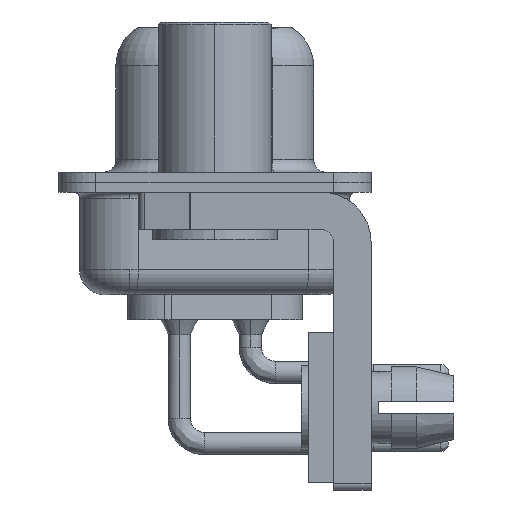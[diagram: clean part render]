
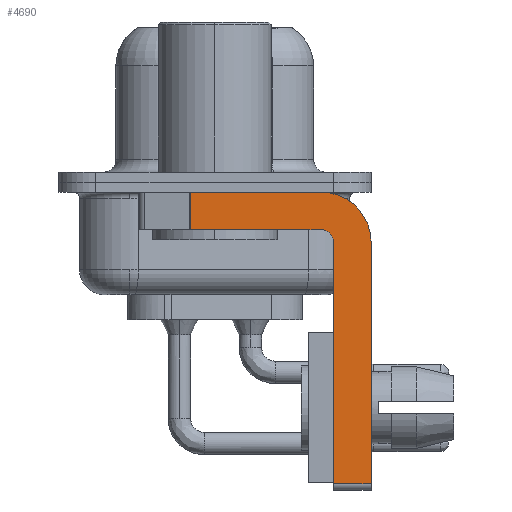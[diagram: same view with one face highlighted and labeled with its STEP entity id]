
A CAD part, left-side view. The second image highlights one B-rep face of the part: STEP entity #4690.
In plain terms, the highlighted planar face has unit normal (-1, 0, 0).
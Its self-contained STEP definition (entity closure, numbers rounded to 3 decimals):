
#132 = CARTESIAN_POINT ( 'NONE',  ( -2.9, -4.25, -1.9 ) ) ;
#850 = CARTESIAN_POINT ( 'NONE',  ( -2.9, -4.25, -1.9 ) ) ;
#1033 = DIRECTION ( 'NONE',  ( -1., 0., 0. ) ) ;
#1676 = LINE ( 'NONE', #17092, #6828 ) ;
#1708 = LINE ( 'NONE', #9999, #8234 ) ;
#1746 = DIRECTION ( 'NONE',  ( 1., 0., 0. ) ) ;
#1796 = CARTESIAN_POINT ( 'NONE',  ( -2.9, 0.978, -1.9 ) ) ;
#1817 = CARTESIAN_POINT ( 'NONE',  ( -2.9, -4.25, -2.4 ) ) ;
#2197 = LINE ( 'NONE', #16255, #24327 ) ;
#2657 = CARTESIAN_POINT ( 'NONE',  ( -2.9, -4.25, -2.4 ) ) ;
#2817 = ORIENTED_EDGE ( 'NONE', *, *, #11641, .F. ) ;
#3050 = EDGE_CURVE ( 'NONE', #20689, #22344, #12436, .T. ) ;
#3237 = LINE ( 'NONE', #25638, #19055 ) ;
#3828 = DIRECTION ( 'NONE',  ( 0., 0., -1. ) ) ;
#3836 = CARTESIAN_POINT ( 'NONE',  ( -2.9, -4.25, -0.4 ) ) ;
#3921 = PLANE ( 'NONE',  #12846 ) ;
#4125 = VERTEX_POINT ( 'NONE', #23902 ) ;
#4253 = EDGE_CURVE ( 'NONE', #18430, #20689, #10383, .T. ) ;
#4690 = ADVANCED_FACE ( 'NONE', ( #8399 ), #3921, .F. ) ;
#4840 = DIRECTION ( 'NONE',  ( 0., 0., -1. ) ) ;
#6702 = CIRCLE ( 'NONE', #15399, 2. ) ;
#6828 = VECTOR ( 'NONE', #14935, 1000. ) ;
#7972 = DIRECTION ( 'NONE',  ( 0., -1., 0. ) ) ;
#8056 = CARTESIAN_POINT ( 'NONE',  ( -2.9, 0.978, -0.4 ) ) ;
#8234 = VECTOR ( 'NONE', #22699, 1000. ) ;
#8399 = FACE_OUTER_BOUND ( 'NONE', #14441, .T. ) ;
#9729 = CARTESIAN_POINT ( 'NONE',  ( -2.9, -4.75, -2.4 ) ) ;
#9807 = DIRECTION ( 'NONE',  ( 0., 0., 1. ) ) ;
#9999 = CARTESIAN_POINT ( 'NONE',  ( -2.9, 0.978, -1.9 ) ) ;
#10218 = CARTESIAN_POINT ( 'NONE',  ( -2.9, -6.25, -12.05 ) ) ;
#10249 = VERTEX_POINT ( 'NONE', #21769 ) ;
#10383 = CIRCLE ( 'NONE', #13934, 0.5 ) ;
#11376 = ORIENTED_EDGE ( 'NONE', *, *, #4253, .F. ) ;
#11641 = EDGE_CURVE ( 'NONE', #10249, #13223, #1676, .T. ) ;
#11762 = VECTOR ( 'NONE', #13123, 1000. ) ;
#12436 = LINE ( 'NONE', #850, #11762 ) ;
#12846 = AXIS2_PLACEMENT_3D ( 'NONE', #1817, #1746, #3828 ) ;
#13085 = ORIENTED_EDGE ( 'NONE', *, *, #18208, .T. ) ;
#13123 = DIRECTION ( 'NONE',  ( 0., 1., 0. ) ) ;
#13223 = VERTEX_POINT ( 'NONE', #10218 ) ;
#13764 = LINE ( 'NONE', #20746, #16429 ) ;
#13934 = AXIS2_PLACEMENT_3D ( 'NONE', #16366, #1033, #22653 ) ;
#14441 = EDGE_LOOP ( 'NONE', ( #15080, #16187, #17750, #11376, #27013, #13085, #2817, #27004 ) ) ;
#14485 = EDGE_CURVE ( 'NONE', #22256, #10249, #6702, .T. ) ;
#14743 = EDGE_CURVE ( 'NONE', #21730, #22256, #13764, .T. ) ;
#14935 = DIRECTION ( 'NONE',  ( 0., 0., -1. ) ) ;
#15080 = ORIENTED_EDGE ( 'NONE', *, *, #14743, .F. ) ;
#15399 = AXIS2_PLACEMENT_3D ( 'NONE', #2657, #17721, #4840 ) ;
#16187 = ORIENTED_EDGE ( 'NONE', *, *, #20414, .T. ) ;
#16255 = CARTESIAN_POINT ( 'NONE',  ( -2.9, -4.75, -12.3 ) ) ;
#16366 = CARTESIAN_POINT ( 'NONE',  ( -2.9, -4.25, -2.4 ) ) ;
#16429 = VECTOR ( 'NONE', #7972, 1000. ) ;
#17092 = CARTESIAN_POINT ( 'NONE',  ( -2.9, -6.25, -2.4 ) ) ;
#17721 = DIRECTION ( 'NONE',  ( 1., 0., 0. ) ) ;
#17750 = ORIENTED_EDGE ( 'NONE', *, *, #3050, .F. ) ;
#17910 = EDGE_CURVE ( 'NONE', #4125, #18430, #2197, .T. ) ;
#18208 = EDGE_CURVE ( 'NONE', #4125, #13223, #3237, .T. ) ;
#18430 = VERTEX_POINT ( 'NONE', #9729 ) ;
#19055 = VECTOR ( 'NONE', #21486, 1000. ) ;
#20414 = EDGE_CURVE ( 'NONE', #21730, #22344, #1708, .T. ) ;
#20689 = VERTEX_POINT ( 'NONE', #132 ) ;
#20746 = CARTESIAN_POINT ( 'NONE',  ( -2.9, 3., -0.4 ) ) ;
#21486 = DIRECTION ( 'NONE',  ( 0., -1., 0. ) ) ;
#21730 = VERTEX_POINT ( 'NONE', #8056 ) ;
#21769 = CARTESIAN_POINT ( 'NONE',  ( -2.9, -6.25, -2.4 ) ) ;
#22256 = VERTEX_POINT ( 'NONE', #3836 ) ;
#22344 = VERTEX_POINT ( 'NONE', #1796 ) ;
#22653 = DIRECTION ( 'NONE',  ( 0., 0., 1. ) ) ;
#22699 = DIRECTION ( 'NONE',  ( 0., 0., -1. ) ) ;
#23902 = CARTESIAN_POINT ( 'NONE',  ( -2.9, -4.75, -12.05 ) ) ;
#24327 = VECTOR ( 'NONE', #9807, 1000. ) ;
#25638 = CARTESIAN_POINT ( 'NONE',  ( -2.9, -4.25, -12.05 ) ) ;
#27004 = ORIENTED_EDGE ( 'NONE', *, *, #14485, .F. ) ;
#27013 = ORIENTED_EDGE ( 'NONE', *, *, #17910, .F. ) ;
